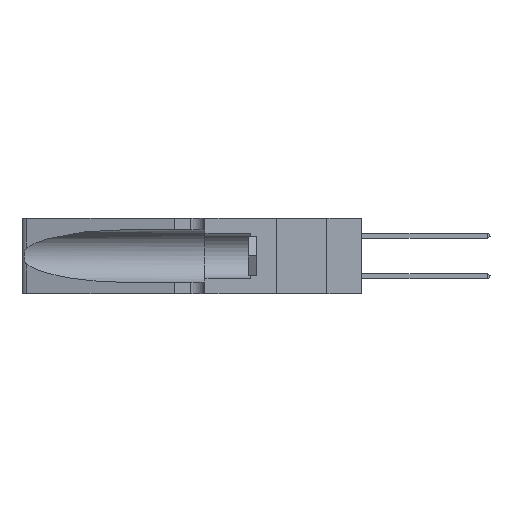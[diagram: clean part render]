
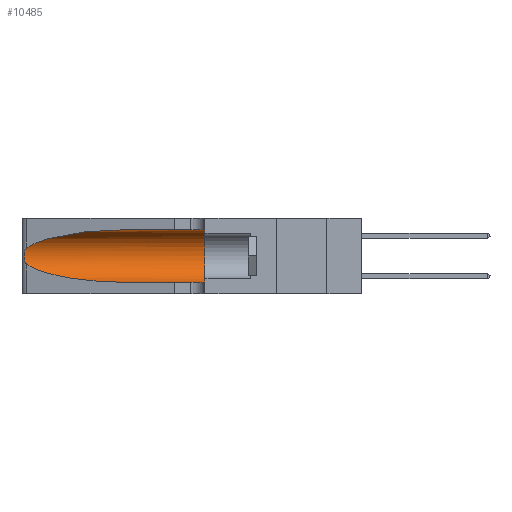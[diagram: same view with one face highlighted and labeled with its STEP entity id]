
A CAD part, left-side view. The second image highlights one B-rep face of the part: STEP entity #10485.
In plain terms, the highlighted cylindrical face has radius 3.308 mm (diameter 6.617 mm), a partial arc.
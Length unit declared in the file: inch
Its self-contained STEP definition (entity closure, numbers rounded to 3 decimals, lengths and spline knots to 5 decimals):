
#72 = VERTEX_POINT ( 'NONE', #5060 ) ;
#817 = CARTESIAN_POINT ( 'NONE',  ( 0.1305, 0.72297, 0.05475 ) ) ;
#1291 = CARTESIAN_POINT ( 'NONE',  ( 0.25555, 1.22993, 0.14849 ) ) ;
#2175 = CARTESIAN_POINT ( 'NONE',  ( 0.1305, 0.72297, 0.31525 ) ) ;
#3211 = CARTESIAN_POINT ( 'NONE',  ( 0.1305, 0.35, 0.185 ) ) ;
#3459 = DIRECTION ( 'NONE',  ( 0., 0., -1. ) ) ;
#3982 = EDGE_CURVE ( 'NONE', #11517, #18112, #33968, .T. ) ;
#4215 = CARTESIAN_POINT ( 'NONE',  ( 0.18966, 0.96281, 0.31525 ) ) ;
#5060 = CARTESIAN_POINT ( 'NONE',  ( 0.25487, 1.22718, 0.22369 ) ) ;
#5095 = CARTESIAN_POINT ( 'NONE',  ( 0.1305, 0.35, 0.31525 ) ) ;
#6528 = EDGE_CURVE ( 'NONE', #11517, #72, #10203, .T. ) ;
#6599 = AXIS2_PLACEMENT_3D ( 'NONE', #3211, #26998, #6691 ) ;
#6691 = DIRECTION ( 'NONE',  ( 0., 0., 1. ) ) ;
#6770 = CYLINDRICAL_SURFACE ( 'NONE', #20850, 0.13025 ) ;
#8101 = CARTESIAN_POINT ( 'NONE',  ( 0.25787, 1.23484, 0.2124 ) ) ;
#8968 = ORIENTED_EDGE ( 'NONE', *, *, #3982, .F. ) ;
#9758 = EDGE_CURVE ( 'NONE', #18112, #39910, #28568, .T. ) ;
#10203 =( BOUNDED_CURVE ( )  B_SPLINE_CURVE ( 3, ( #41235, #4215, #41369, #21362 ),
 .UNSPECIFIED., .F., .F. ) 
 B_SPLINE_CURVE_WITH_KNOTS ( ( 4, 4 ),
 ( 1.5708, 2.84003 ),
 .UNSPECIFIED. ) 
 CURVE ( )  GEOMETRIC_REPRESENTATION_ITEM ( )  RATIONAL_B_SPLINE_CURVE ( ( 1., 0.87, 0.87, 1. ) ) 
 REPRESENTATION_ITEM ( '' )  );
#10485 = ADVANCED_FACE ( 'NONE', ( #42551 ), #6770, .F. ) ;
#10588 = CARTESIAN_POINT ( 'NONE',  ( 0.1305, 1.61858, 0.31525 ) ) ;
#11197 = VERTEX_POINT ( 'NONE', #817 ) ;
#11517 = VERTEX_POINT ( 'NONE', #2175 ) ;
#11561 = CARTESIAN_POINT ( 'NONE',  ( 0.26018, 1.23835, 0.19895 ) ) ;
#11692 = LINE ( 'NONE', #31570, #18578 ) ;
#14001 = DIRECTION ( 'NONE',  ( 0., -1., 0. ) ) ;
#14080 = VERTEX_POINT ( 'NONE', #43549 ) ;
#14946 = CARTESIAN_POINT ( 'NONE',  ( 0.26075, 1.23896, 0.178 ) ) ;
#16386 = CARTESIAN_POINT ( 'NONE',  ( 0.25487, 1.22718, 0.14631 ) ) ;
#16973 = ORIENTED_EDGE ( 'NONE', *, *, #6528, .T. ) ;
#18016 = EDGE_CURVE ( 'NONE', #72, #14080, #30487, .T. ) ;
#18112 = VERTEX_POINT ( 'NONE', #5095 ) ;
#18369 = CARTESIAN_POINT ( 'NONE',  ( 0.25856, 1.23593, 0.16098 ) ) ;
#18578 = VECTOR ( 'NONE', #34923, 39.37008 ) ;
#19581 = ORIENTED_EDGE ( 'NONE', *, *, #18016, .T. ) ;
#19798 = CARTESIAN_POINT ( 'NONE',  ( 0.2373, 1.15595, 0.08982 ) ) ;
#20446 = DIRECTION ( 'NONE',  ( 0., -1., 0. ) ) ;
#20613 = ORIENTED_EDGE ( 'NONE', *, *, #32451, .T. ) ;
#20850 = AXIS2_PLACEMENT_3D ( 'NONE', #30596, #20446, #3459 ) ;
#21362 = CARTESIAN_POINT ( 'NONE',  ( 0.25487, 1.22718, 0.22369 ) ) ;
#21750 = CARTESIAN_POINT ( 'NONE',  ( 0.25639, 1.23186, 0.15144 ) ) ;
#22757 = ORIENTED_EDGE ( 'NONE', *, *, #32114, .T. ) ;
#23213 = CARTESIAN_POINT ( 'NONE',  ( 0.1305, 0.72297, 0.05475 ) ) ;
#25152 = CARTESIAN_POINT ( 'NONE',  ( 0.25487, 1.22718, 0.14631 ) ) ;
#26998 = DIRECTION ( 'NONE',  ( 0., 1., 0. ) ) ;
#27225 = EDGE_LOOP ( 'NONE', ( #16973, #19581, #20613, #22757, #40517, #8968 ) ) ;
#27274 =( BOUNDED_CURVE ( )  B_SPLINE_CURVE ( 3, ( #16386, #19798, #43168, #23213 ),
 .UNSPECIFIED., .F., .T. ) 
 B_SPLINE_CURVE_WITH_KNOTS ( ( 4, 4 ),
 ( 3.44316, 4.71239 ),
 .UNSPECIFIED. ) 
 CURVE ( )  GEOMETRIC_REPRESENTATION_ITEM ( )  RATIONAL_B_SPLINE_CURVE ( ( 1., 0.87, 0.87, 1. ) ) 
 REPRESENTATION_ITEM ( '' )  );
#27836 = CARTESIAN_POINT ( 'NONE',  ( 0.1305, 0.35, 0.05475 ) ) ;
#28380 = CARTESIAN_POINT ( 'NONE',  ( 0.25639, 1.23184, 0.21858 ) ) ;
#28568 = CIRCLE ( 'NONE', #6599, 0.13025 ) ;
#30487 = B_SPLINE_CURVE_WITH_KNOTS ( 'NONE', 3,
 ( #38287, #41468, #28380, #8101, #31739, #11561, #35089, #14946, #38431, #18369, #41747, #21750, #1291, #25152 ),
 .UNSPECIFIED., .F., .F.,
 ( 4, 2, 2, 2, 2, 2, 4 ),
 ( 0., 0.00027, 0.00053, 0.00107, 0.0016, 0.00187, 0.00214 ),
 .UNSPECIFIED. ) ;
#30596 = CARTESIAN_POINT ( 'NONE',  ( 0.1305, 1.61858, 0.185 ) ) ;
#31570 = CARTESIAN_POINT ( 'NONE',  ( 0.1305, 1.61858, 0.05475 ) ) ;
#31739 = CARTESIAN_POINT ( 'NONE',  ( 0.25854, 1.2359, 0.20912 ) ) ;
#32114 = EDGE_CURVE ( 'NONE', #11197, #39910, #11692, .T. ) ;
#32451 = EDGE_CURVE ( 'NONE', #14080, #11197, #27274, .T. ) ;
#33968 = LINE ( 'NONE', #10588, #40723 ) ;
#34923 = DIRECTION ( 'NONE',  ( 0., -1., 0. ) ) ;
#35089 = CARTESIAN_POINT ( 'NONE',  ( 0.26075, 1.23896, 0.19203 ) ) ;
#38287 = CARTESIAN_POINT ( 'NONE',  ( 0.25487, 1.22718, 0.22369 ) ) ;
#38431 = CARTESIAN_POINT ( 'NONE',  ( 0.26017, 1.23833, 0.17102 ) ) ;
#39910 = VERTEX_POINT ( 'NONE', #27836 ) ;
#40517 = ORIENTED_EDGE ( 'NONE', *, *, #9758, .F. ) ;
#40723 = VECTOR ( 'NONE', #14001, 39.37008 ) ;
#41235 = CARTESIAN_POINT ( 'NONE',  ( 0.1305, 0.72297, 0.31525 ) ) ;
#41369 = CARTESIAN_POINT ( 'NONE',  ( 0.2373, 1.15595, 0.28018 ) ) ;
#41468 = CARTESIAN_POINT ( 'NONE',  ( 0.25555, 1.22994, 0.2215 ) ) ;
#41747 = CARTESIAN_POINT ( 'NONE',  ( 0.25789, 1.23486, 0.15765 ) ) ;
#42551 = FACE_OUTER_BOUND ( 'NONE', #27225, .T. ) ;
#43168 = CARTESIAN_POINT ( 'NONE',  ( 0.18966, 0.96281, 0.05475 ) ) ;
#43549 = CARTESIAN_POINT ( 'NONE',  ( 0.25487, 1.22718, 0.14631 ) ) ;
